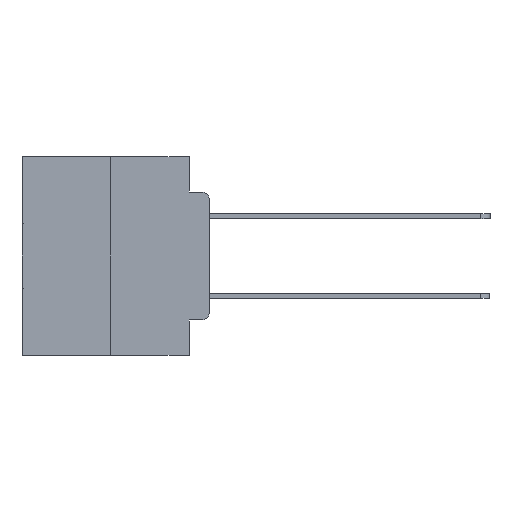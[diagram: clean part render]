
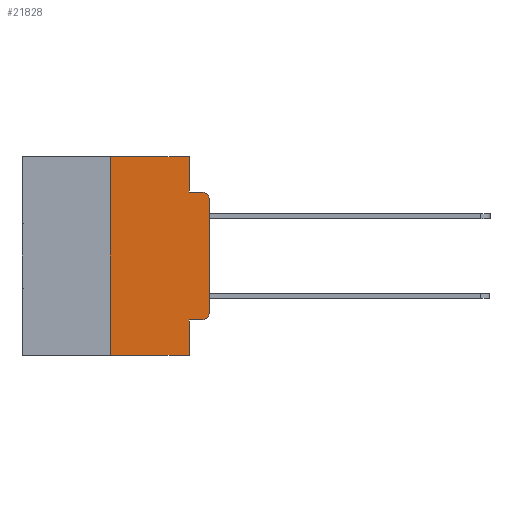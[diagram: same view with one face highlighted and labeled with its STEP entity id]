
A CAD part, left-side view. The second image highlights one B-rep face of the part: STEP entity #21828.
In plain terms, the highlighted planar face has unit normal (-1, 0, 0).
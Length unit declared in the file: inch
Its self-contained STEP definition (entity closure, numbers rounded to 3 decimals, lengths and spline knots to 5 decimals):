
#168 = ORIENTED_EDGE ( 'NONE', *, *, #13315, .T. ) ;
#644 = ORIENTED_EDGE ( 'NONE', *, *, #4549, .F. ) ;
#710 = AXIS2_PLACEMENT_3D ( 'NONE', #15519, #6079, #22782 ) ;
#919 = LINE ( 'NONE', #20727, #2474 ) ;
#1230 = CARTESIAN_POINT ( 'NONE',  ( 0., 0.051, -0.4115 ) ) ;
#1500 = DIRECTION ( 'NONE',  ( 0., 0., -1. ) ) ;
#1582 = DIRECTION ( 'NONE',  ( 0., 0., 1. ) ) ;
#1847 = DIRECTION ( 'NONE',  ( 0., 0., -1. ) ) ;
#2455 = EDGE_CURVE ( 'NONE', #10720, #9280, #919, .T. ) ;
#2474 = VECTOR ( 'NONE', #4018, 39.37008 ) ;
#2685 = EDGE_CURVE ( 'NONE', #24976, #15671, #25953, .T. ) ;
#2795 = CARTESIAN_POINT ( 'NONE',  ( 0., 0.051, 0. ) ) ;
#2934 = ORIENTED_EDGE ( 'NONE', *, *, #17097, .T. ) ;
#3174 = VECTOR ( 'NONE', #7380, 39.37008 ) ;
#4018 = DIRECTION ( 'NONE',  ( 0., -1., 0. ) ) ;
#4036 = CARTESIAN_POINT ( 'NONE',  ( 0., 0.25, -0.5 ) ) ;
#4162 = ORIENTED_EDGE ( 'NONE', *, *, #2685, .F. ) ;
#4496 = LINE ( 'NONE', #30675, #10078 ) ;
#4549 = EDGE_CURVE ( 'NONE', #9492, #11661, #4496, .T. ) ;
#5246 = FACE_OUTER_BOUND ( 'NONE', #30812, .T. ) ;
#5330 = EDGE_CURVE ( 'NONE', #11661, #24976, #18613, .T. ) ;
#5569 = CARTESIAN_POINT ( 'NONE',  ( 0., 0.051, -0.5 ) ) ;
#6079 = DIRECTION ( 'NONE',  ( 1., 0., 0. ) ) ;
#6228 = ORIENTED_EDGE ( 'NONE', *, *, #25076, .F. ) ;
#6526 = EDGE_CURVE ( 'NONE', #17359, #7057, #22267, .T. ) ;
#6949 = CARTESIAN_POINT ( 'NONE',  ( 0., 0.02, -0.4115 ) ) ;
#7057 = VERTEX_POINT ( 'NONE', #23721 ) ;
#7062 = ORIENTED_EDGE ( 'NONE', *, *, #26064, .F. ) ;
#7162 = CARTESIAN_POINT ( 'NONE',  ( 0., 0.051, 0. ) ) ;
#7380 = DIRECTION ( 'NONE',  ( 0., 0., 1. ) ) ;
#8016 = VECTOR ( 'NONE', #1582, 39.37008 ) ;
#8263 = AXIS2_PLACEMENT_3D ( 'NONE', #30353, #16163, #1847 ) ;
#9280 = VERTEX_POINT ( 'NONE', #5569 ) ;
#9492 = VERTEX_POINT ( 'NONE', #23009 ) ;
#9546 = EDGE_CURVE ( 'NONE', #25869, #17359, #26861, .T. ) ;
#9770 = CARTESIAN_POINT ( 'NONE',  ( 0., 0., 0. ) ) ;
#10078 = VECTOR ( 'NONE', #18927, 39.37008 ) ;
#10540 = LINE ( 'NONE', #30130, #28727 ) ;
#10720 = VERTEX_POINT ( 'NONE', #4036 ) ;
#10804 = DIRECTION ( 'NONE',  ( 0., -1., 0. ) ) ;
#11661 = VERTEX_POINT ( 'NONE', #7162 ) ;
#12508 = AXIS2_PLACEMENT_3D ( 'NONE', #28062, #13879, #30438 ) ;
#13312 = VECTOR ( 'NONE', #16800, 39.37008 ) ;
#13315 = EDGE_CURVE ( 'NONE', #18845, #25869, #13383, .T. ) ;
#13383 = LINE ( 'NONE', #1230, #18975 ) ;
#13879 = DIRECTION ( 'NONE',  ( -1., 0., 0. ) ) ;
#14210 = CARTESIAN_POINT ( 'NONE',  ( 0., 0.051, -0.0885 ) ) ;
#14333 = LINE ( 'NONE', #30107, #8016 ) ;
#14864 = ORIENTED_EDGE ( 'NONE', *, *, #5330, .F. ) ;
#15519 = CARTESIAN_POINT ( 'NONE',  ( 0., 0.473, 0. ) ) ;
#15671 = VERTEX_POINT ( 'NONE', #20696 ) ;
#16163 = DIRECTION ( 'NONE',  ( -1., 0., 0. ) ) ;
#16800 = DIRECTION ( 'NONE',  ( 0., -1., 0. ) ) ;
#17097 = EDGE_CURVE ( 'NONE', #7057, #15671, #22683, .T. ) ;
#17104 = DIRECTION ( 'NONE',  ( 0., 0., -1. ) ) ;
#17359 = VERTEX_POINT ( 'NONE', #24094 ) ;
#18417 = ORIENTED_EDGE ( 'NONE', *, *, #2455, .T. ) ;
#18613 = LINE ( 'NONE', #2795, #25663 ) ;
#18845 = VERTEX_POINT ( 'NONE', #22997 ) ;
#18927 = DIRECTION ( 'NONE',  ( 0., -1., 0. ) ) ;
#18975 = VECTOR ( 'NONE', #10804, 39.37008 ) ;
#20232 = CARTESIAN_POINT ( 'NONE',  ( 0., 0.051, -0.0885 ) ) ;
#20696 = CARTESIAN_POINT ( 'NONE',  ( 0., 0.02, -0.0885 ) ) ;
#20727 = CARTESIAN_POINT ( 'NONE',  ( 0., 0.473, -0.5 ) ) ;
#21227 = ORIENTED_EDGE ( 'NONE', *, *, #6526, .T. ) ;
#21828 = ADVANCED_FACE ( 'NONE', ( #5246 ), #25023, .F. ) ;
#22267 = LINE ( 'NONE', #9770, #3174 ) ;
#22683 = CIRCLE ( 'NONE', #12508, 0.02 ) ;
#22782 = DIRECTION ( 'NONE',  ( 0., 0., -1. ) ) ;
#22997 = CARTESIAN_POINT ( 'NONE',  ( 0., 0.051, -0.4115 ) ) ;
#23009 = CARTESIAN_POINT ( 'NONE',  ( 0., 0.25, 0. ) ) ;
#23721 = CARTESIAN_POINT ( 'NONE',  ( 0., 0., -0.1085 ) ) ;
#24094 = CARTESIAN_POINT ( 'NONE',  ( 0., 0., -0.3915 ) ) ;
#24621 = ORIENTED_EDGE ( 'NONE', *, *, #9546, .T. ) ;
#24976 = VERTEX_POINT ( 'NONE', #20232 ) ;
#25023 = PLANE ( 'NONE',  #710 ) ;
#25076 = EDGE_CURVE ( 'NONE', #10720, #9492, #14333, .T. ) ;
#25663 = VECTOR ( 'NONE', #17104, 39.37008 ) ;
#25869 = VERTEX_POINT ( 'NONE', #6949 ) ;
#25953 = LINE ( 'NONE', #14210, #13312 ) ;
#26064 = EDGE_CURVE ( 'NONE', #18845, #9280, #10540, .T. ) ;
#26861 = CIRCLE ( 'NONE', #8263, 0.02 ) ;
#28062 = CARTESIAN_POINT ( 'NONE',  ( 0., 0.02, -0.1085 ) ) ;
#28727 = VECTOR ( 'NONE', #1500, 39.37008 ) ;
#30107 = CARTESIAN_POINT ( 'NONE',  ( 0., 0.25, 0. ) ) ;
#30130 = CARTESIAN_POINT ( 'NONE',  ( 0., 0.051, 0. ) ) ;
#30353 = CARTESIAN_POINT ( 'NONE',  ( 0., 0.02, -0.3915 ) ) ;
#30438 = DIRECTION ( 'NONE',  ( 0., 0., -1. ) ) ;
#30675 = CARTESIAN_POINT ( 'NONE',  ( 0., 0.473, 0. ) ) ;
#30812 = EDGE_LOOP ( 'NONE', ( #21227, #2934, #4162, #14864, #644, #6228, #18417, #7062, #168, #24621 ) ) ;
